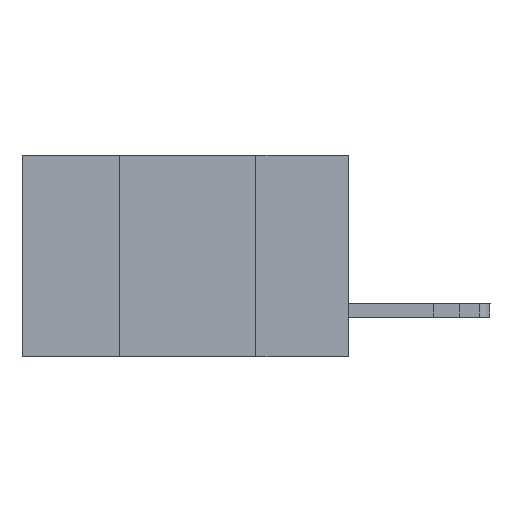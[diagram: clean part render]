
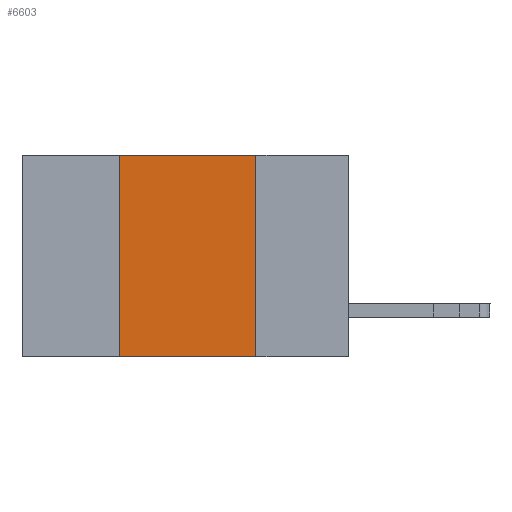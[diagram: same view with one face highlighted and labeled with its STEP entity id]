
A CAD part, left-side view. The second image highlights one B-rep face of the part: STEP entity #6603.
In plain terms, the highlighted planar face has unit normal (-1, 0, 0).
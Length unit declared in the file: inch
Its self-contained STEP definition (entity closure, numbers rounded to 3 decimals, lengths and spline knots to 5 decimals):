
#65 = VECTOR ( 'NONE', #867, 39.37008 ) ;
#70 = ORIENTED_EDGE ( 'NONE', *, *, #675, .F. ) ;
#198 = VECTOR ( 'NONE', #11286, 39.37008 ) ;
#225 = CARTESIAN_POINT ( 'NONE',  ( 0., 0.6, 0. ) ) ;
#334 = AXIS2_PLACEMENT_3D ( 'NONE', #225, #2678, #864 ) ;
#437 = CARTESIAN_POINT ( 'NONE',  ( 0., 0.17, -0.37 ) ) ;
#538 = VERTEX_POINT ( 'NONE', #6675 ) ;
#673 = EDGE_CURVE ( 'NONE', #2807, #9349, #2607, .T. ) ;
#675 = EDGE_CURVE ( 'NONE', #538, #7196, #2663, .T. ) ;
#864 = DIRECTION ( 'NONE',  ( 0., 0., -1. ) ) ;
#867 = DIRECTION ( 'NONE',  ( 0., -1., 0. ) ) ;
#1806 = CARTESIAN_POINT ( 'NONE',  ( 0., 0.17, -0.37 ) ) ;
#1951 = CARTESIAN_POINT ( 'NONE',  ( 0., 0.42, 0. ) ) ;
#2607 = LINE ( 'NONE', #5170, #198 ) ;
#2663 = LINE ( 'NONE', #1806, #10598 ) ;
#2678 = DIRECTION ( 'NONE',  ( 1., 0., 0. ) ) ;
#2807 = VERTEX_POINT ( 'NONE', #7725 ) ;
#4102 = EDGE_CURVE ( 'NONE', #9349, #538, #9056, .T. ) ;
#4198 = CARTESIAN_POINT ( 'NONE',  ( 0., 0.6, -0.37 ) ) ;
#4369 = EDGE_CURVE ( 'NONE', #2807, #7196, #9518, .T. ) ;
#4514 = PLANE ( 'NONE',  #334 ) ;
#4523 = EDGE_LOOP ( 'NONE', ( #70, #10696, #6315, #4748 ) ) ;
#4748 = ORIENTED_EDGE ( 'NONE', *, *, #4369, .T. ) ;
#4758 = CARTESIAN_POINT ( 'NONE',  ( 0., 0.6, 0. ) ) ;
#5170 = CARTESIAN_POINT ( 'NONE',  ( 0., 0.42, -0.37 ) ) ;
#5372 = DIRECTION ( 'NONE',  ( 0., -1., 0. ) ) ;
#5881 = VECTOR ( 'NONE', #5372, 39.37008 ) ;
#6315 = ORIENTED_EDGE ( 'NONE', *, *, #673, .F. ) ;
#6603 = ADVANCED_FACE ( 'NONE', ( #9679 ), #4514, .F. ) ;
#6675 = CARTESIAN_POINT ( 'NONE',  ( 0., 0.17, 0. ) ) ;
#7196 = VERTEX_POINT ( 'NONE', #437 ) ;
#7725 = CARTESIAN_POINT ( 'NONE',  ( 0., 0.42, -0.37 ) ) ;
#9017 = DIRECTION ( 'NONE',  ( 0., 0., -1. ) ) ;
#9056 = LINE ( 'NONE', #4758, #5881 ) ;
#9349 = VERTEX_POINT ( 'NONE', #1951 ) ;
#9518 = LINE ( 'NONE', #4198, #65 ) ;
#9679 = FACE_OUTER_BOUND ( 'NONE', #4523, .T. ) ;
#10598 = VECTOR ( 'NONE', #9017, 39.37008 ) ;
#10696 = ORIENTED_EDGE ( 'NONE', *, *, #4102, .F. ) ;
#11286 = DIRECTION ( 'NONE',  ( 0., 0., 1. ) ) ;
